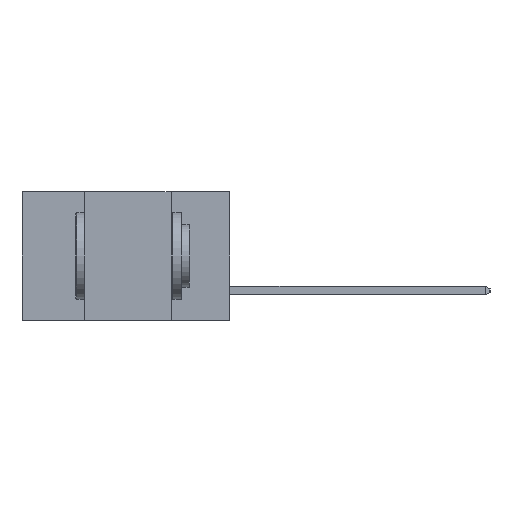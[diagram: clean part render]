
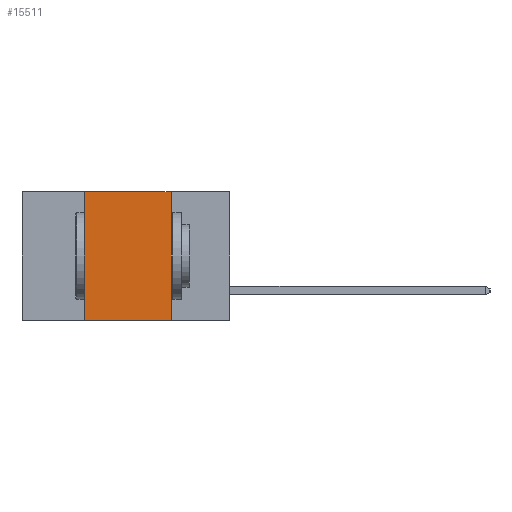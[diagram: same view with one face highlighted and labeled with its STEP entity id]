
A CAD part, left-side view. The second image highlights one B-rep face of the part: STEP entity #15511.
In plain terms, the highlighted planar face has unit normal (-1, 0, 0).
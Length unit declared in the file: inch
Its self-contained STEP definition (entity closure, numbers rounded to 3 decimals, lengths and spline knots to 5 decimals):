
#462 = DIRECTION ( 'NONE',  ( 0., 0., -1. ) ) ;
#1258 = ORIENTED_EDGE ( 'NONE', *, *, #16231, .F. ) ;
#2122 = CARTESIAN_POINT ( 'NONE',  ( 0., 0.6, 0. ) ) ;
#2319 = CARTESIAN_POINT ( 'NONE',  ( 0., 0.42, -0.37 ) ) ;
#3179 = LINE ( 'NONE', #17036, #17685 ) ;
#4036 = DIRECTION ( 'NONE',  ( 0., 0., -1. ) ) ;
#6717 = CARTESIAN_POINT ( 'NONE',  ( 0., 0.17, 0. ) ) ;
#6911 = EDGE_CURVE ( 'NONE', #16750, #7595, #15650, .T. ) ;
#7479 = EDGE_CURVE ( 'NONE', #20201, #8812, #22415, .T. ) ;
#7595 = VERTEX_POINT ( 'NONE', #20309 ) ;
#7913 = FACE_OUTER_BOUND ( 'NONE', #19827, .T. ) ;
#8157 = ORIENTED_EDGE ( 'NONE', *, *, #7479, .F. ) ;
#8812 = VERTEX_POINT ( 'NONE', #6717 ) ;
#10651 = VECTOR ( 'NONE', #11472, 39.37008 ) ;
#11421 = VECTOR ( 'NONE', #462, 39.37008 ) ;
#11455 = DIRECTION ( 'NONE',  ( 0., 0., 1. ) ) ;
#11472 = DIRECTION ( 'NONE',  ( 0., -1., 0. ) ) ;
#12020 = LINE ( 'NONE', #23065, #11421 ) ;
#12314 = ORIENTED_EDGE ( 'NONE', *, *, #6911, .T. ) ;
#14818 = CARTESIAN_POINT ( 'NONE',  ( 0., 0.6, -0.37 ) ) ;
#14891 = AXIS2_PLACEMENT_3D ( 'NONE', #2122, #15397, #4036 ) ;
#15397 = DIRECTION ( 'NONE',  ( 1., 0., 0. ) ) ;
#15511 = ADVANCED_FACE ( 'NONE', ( #7913 ), #22783, .F. ) ;
#15650 = LINE ( 'NONE', #14818, #10651 ) ;
#16231 = EDGE_CURVE ( 'NONE', #8812, #7595, #12020, .T. ) ;
#16750 = VERTEX_POINT ( 'NONE', #2319 ) ;
#16897 = VECTOR ( 'NONE', #19726, 39.37008 ) ;
#17036 = CARTESIAN_POINT ( 'NONE',  ( 0., 0.42, 0. ) ) ;
#17685 = VECTOR ( 'NONE', #11455, 39.37008 ) ;
#19438 = CARTESIAN_POINT ( 'NONE',  ( 0., 0.6, 0. ) ) ;
#19726 = DIRECTION ( 'NONE',  ( 0., -1., 0. ) ) ;
#19827 = EDGE_LOOP ( 'NONE', ( #1258, #8157, #19912, #12314 ) ) ;
#19912 = ORIENTED_EDGE ( 'NONE', *, *, #23845, .F. ) ;
#20201 = VERTEX_POINT ( 'NONE', #24103 ) ;
#20309 = CARTESIAN_POINT ( 'NONE',  ( 0., 0.17, -0.37 ) ) ;
#22415 = LINE ( 'NONE', #19438, #16897 ) ;
#22783 = PLANE ( 'NONE',  #14891 ) ;
#23065 = CARTESIAN_POINT ( 'NONE',  ( 0., 0.17, 0. ) ) ;
#23845 = EDGE_CURVE ( 'NONE', #16750, #20201, #3179, .T. ) ;
#24103 = CARTESIAN_POINT ( 'NONE',  ( 0., 0.42, 0. ) ) ;
